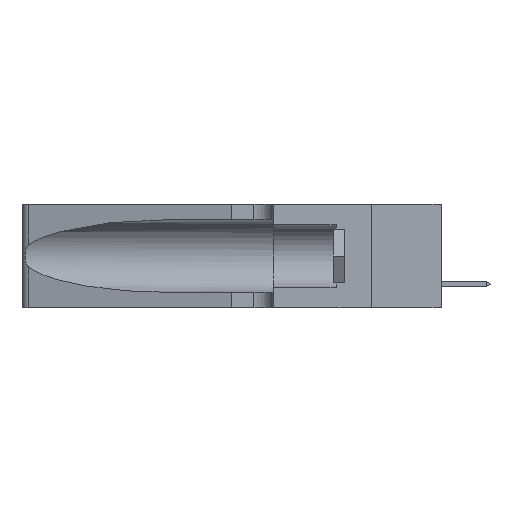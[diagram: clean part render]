
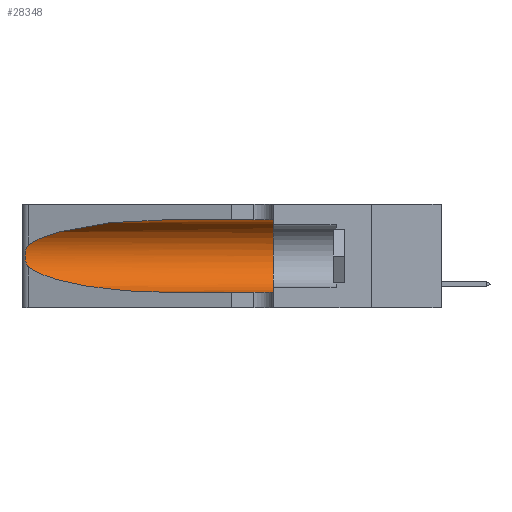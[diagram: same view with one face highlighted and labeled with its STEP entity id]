
A CAD part, left-side view. The second image highlights one B-rep face of the part: STEP entity #28348.
In plain terms, the highlighted cylindrical face has radius 3.308 mm (diameter 6.617 mm), a partial arc.
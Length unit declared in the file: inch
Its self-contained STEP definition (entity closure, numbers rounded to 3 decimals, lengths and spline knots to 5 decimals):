
#13 = FACE_OUTER_BOUND ( 'NONE', #33448, .T. ) ;
#1463 = DIRECTION ( 'NONE',  ( 0., 0., -1. ) ) ;
#1940 = CARTESIAN_POINT ( 'NONE',  ( 0.25854, 1.2359, 0.20912 ) ) ;
#2421 = CARTESIAN_POINT ( 'NONE',  ( 0.25555, 1.22994, 0.2215 ) ) ;
#2465 = VERTEX_POINT ( 'NONE', #4445 ) ;
#3041 = CARTESIAN_POINT ( 'NONE',  ( 0.1305, 1.61858, 0.05475 ) ) ;
#3530 = VERTEX_POINT ( 'NONE', #32602 ) ;
#3909 = CARTESIAN_POINT ( 'NONE',  ( 0.2373, 1.15595, 0.28018 ) ) ;
#4006 = CARTESIAN_POINT ( 'NONE',  ( 0.26018, 1.23835, 0.19895 ) ) ;
#4135 = CARTESIAN_POINT ( 'NONE',  ( 0.2373, 1.15595, 0.08982 ) ) ;
#4445 = CARTESIAN_POINT ( 'NONE',  ( 0.25487, 1.22718, 0.22369 ) ) ;
#5162 = CARTESIAN_POINT ( 'NONE',  ( 0.25639, 1.23184, 0.21858 ) ) ;
#5316 = ORIENTED_EDGE ( 'NONE', *, *, #13170, .F. ) ;
#5794 = CARTESIAN_POINT ( 'NONE',  ( 0.1305, 0.35, 0.31525 ) ) ;
#6067 =( BOUNDED_CURVE ( )  B_SPLINE_CURVE ( 3, ( #9361, #4135, #14699, #19893 ),
 .UNSPECIFIED., .F., .F. ) 
 B_SPLINE_CURVE_WITH_KNOTS ( ( 4, 4 ),
 ( 3.44316, 4.71239 ),
 .UNSPECIFIED. ) 
 CURVE ( )  GEOMETRIC_REPRESENTATION_ITEM ( )  RATIONAL_B_SPLINE_CURVE ( ( 1., 0.87, 0.87, 1. ) ) 
 REPRESENTATION_ITEM ( '' )  );
#6106 = DIRECTION ( 'NONE',  ( 0., -1., 0. ) ) ;
#6448 = AXIS2_PLACEMENT_3D ( 'NONE', #30515, #17384, #14957 ) ;
#6611 = CARTESIAN_POINT ( 'NONE',  ( 0.25487, 1.22718, 0.22369 ) ) ;
#8706 = CARTESIAN_POINT ( 'NONE',  ( 0.25555, 1.22993, 0.14849 ) ) ;
#9361 = CARTESIAN_POINT ( 'NONE',  ( 0.25487, 1.22718, 0.14631 ) ) ;
#10221 = DIRECTION ( 'NONE',  ( 0., -1., 0. ) ) ;
#10930 = EDGE_CURVE ( 'NONE', #19079, #3530, #32047, .T. ) ;
#11134 = CARTESIAN_POINT ( 'NONE',  ( 0.26075, 1.23896, 0.19203 ) ) ;
#11702 = ORIENTED_EDGE ( 'NONE', *, *, #10930, .T. ) ;
#11941 = CARTESIAN_POINT ( 'NONE',  ( 0.1305, 1.61858, 0.31525 ) ) ;
#13010 = EDGE_CURVE ( 'NONE', #17211, #19079, #6067, .T. ) ;
#13170 = EDGE_CURVE ( 'NONE', #21169, #33694, #25678, .T. ) ;
#13919 = CARTESIAN_POINT ( 'NONE',  ( 0.25789, 1.23486, 0.15765 ) ) ;
#14699 = CARTESIAN_POINT ( 'NONE',  ( 0.18966, 0.96281, 0.05475 ) ) ;
#14957 = DIRECTION ( 'NONE',  ( 0., 0., 1. ) ) ;
#16293 = CARTESIAN_POINT ( 'NONE',  ( 0.1305, 0.72297, 0.31525 ) ) ;
#16690 = CARTESIAN_POINT ( 'NONE',  ( 0.25487, 1.22718, 0.14631 ) ) ;
#17151 = CARTESIAN_POINT ( 'NONE',  ( 0.18966, 0.96281, 0.31525 ) ) ;
#17211 = VERTEX_POINT ( 'NONE', #16690 ) ;
#17353 = VECTOR ( 'NONE', #10221, 39.37008 ) ;
#17384 = DIRECTION ( 'NONE',  ( 0., 1., 0. ) ) ;
#17469 = EDGE_CURVE ( 'NONE', #21169, #2465, #24130, .T. ) ;
#17968 = EDGE_CURVE ( 'NONE', #2465, #17211, #17989, .T. ) ;
#17989 = B_SPLINE_CURVE_WITH_KNOTS ( 'NONE', 3,
 ( #18858, #2421, #5162, #24119, #1940, #4006, #11134, #32098, #29501, #24482, #13919, #21879, #8706, #26018 ),
 .UNSPECIFIED., .F., .F.,
 ( 4, 2, 2, 2, 2, 2, 4 ),
 ( 0., 0.00027, 0.00053, 0.00107, 0.0016, 0.00187, 0.00214 ),
 .UNSPECIFIED. ) ;
#18281 = ORIENTED_EDGE ( 'NONE', *, *, #17968, .T. ) ;
#18858 = CARTESIAN_POINT ( 'NONE',  ( 0.25487, 1.22718, 0.22369 ) ) ;
#19079 = VERTEX_POINT ( 'NONE', #33158 ) ;
#19560 = CARTESIAN_POINT ( 'NONE',  ( 0.1305, 0.72297, 0.31525 ) ) ;
#19738 = ORIENTED_EDGE ( 'NONE', *, *, #17469, .T. ) ;
#19893 = CARTESIAN_POINT ( 'NONE',  ( 0.1305, 0.72297, 0.05475 ) ) ;
#21148 = DIRECTION ( 'NONE',  ( 0., -1., 0. ) ) ;
#21169 = VERTEX_POINT ( 'NONE', #16293 ) ;
#21879 = CARTESIAN_POINT ( 'NONE',  ( 0.25639, 1.23186, 0.15144 ) ) ;
#22370 = CYLINDRICAL_SURFACE ( 'NONE', #29983, 0.13025 ) ;
#22385 = ORIENTED_EDGE ( 'NONE', *, *, #13010, .T. ) ;
#23898 = CIRCLE ( 'NONE', #6448, 0.13025 ) ;
#24119 = CARTESIAN_POINT ( 'NONE',  ( 0.25787, 1.23484, 0.2124 ) ) ;
#24130 =( BOUNDED_CURVE ( )  B_SPLINE_CURVE ( 3, ( #19560, #17151, #3909, #6611 ),
 .UNSPECIFIED., .F., .F. ) 
 B_SPLINE_CURVE_WITH_KNOTS ( ( 4, 4 ),
 ( 1.5708, 2.84003 ),
 .UNSPECIFIED. ) 
 CURVE ( )  GEOMETRIC_REPRESENTATION_ITEM ( )  RATIONAL_B_SPLINE_CURVE ( ( 1., 0.87, 0.87, 1. ) ) 
 REPRESENTATION_ITEM ( '' )  );
#24482 = CARTESIAN_POINT ( 'NONE',  ( 0.25856, 1.23593, 0.16098 ) ) ;
#25678 = LINE ( 'NONE', #11941, #17353 ) ;
#26018 = CARTESIAN_POINT ( 'NONE',  ( 0.25487, 1.22718, 0.14631 ) ) ;
#27579 = CARTESIAN_POINT ( 'NONE',  ( 0.1305, 1.61858, 0.185 ) ) ;
#28124 = ORIENTED_EDGE ( 'NONE', *, *, #29448, .F. ) ;
#28348 = ADVANCED_FACE ( 'NONE', ( #13 ), #22370, .F. ) ;
#28713 = VECTOR ( 'NONE', #21148, 39.37008 ) ;
#29448 = EDGE_CURVE ( 'NONE', #33694, #3530, #23898, .T. ) ;
#29501 = CARTESIAN_POINT ( 'NONE',  ( 0.26017, 1.23833, 0.17102 ) ) ;
#29983 = AXIS2_PLACEMENT_3D ( 'NONE', #27579, #6106, #1463 ) ;
#30515 = CARTESIAN_POINT ( 'NONE',  ( 0.1305, 0.35, 0.185 ) ) ;
#32047 = LINE ( 'NONE', #3041, #28713 ) ;
#32098 = CARTESIAN_POINT ( 'NONE',  ( 0.26075, 1.23896, 0.178 ) ) ;
#32602 = CARTESIAN_POINT ( 'NONE',  ( 0.1305, 0.35, 0.05475 ) ) ;
#33158 = CARTESIAN_POINT ( 'NONE',  ( 0.1305, 0.72297, 0.05475 ) ) ;
#33448 = EDGE_LOOP ( 'NONE', ( #19738, #18281, #22385, #11702, #28124, #5316 ) ) ;
#33694 = VERTEX_POINT ( 'NONE', #5794 ) ;
